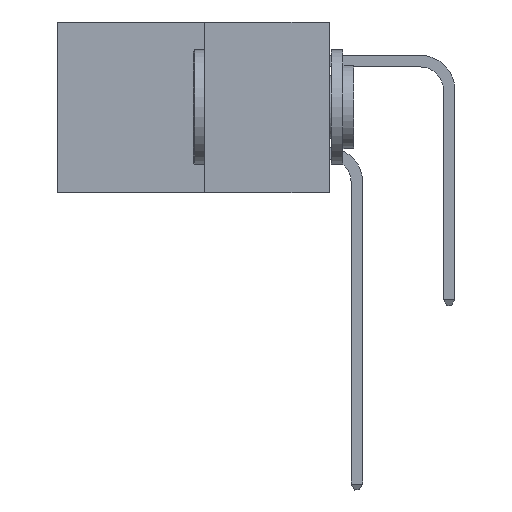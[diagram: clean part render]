
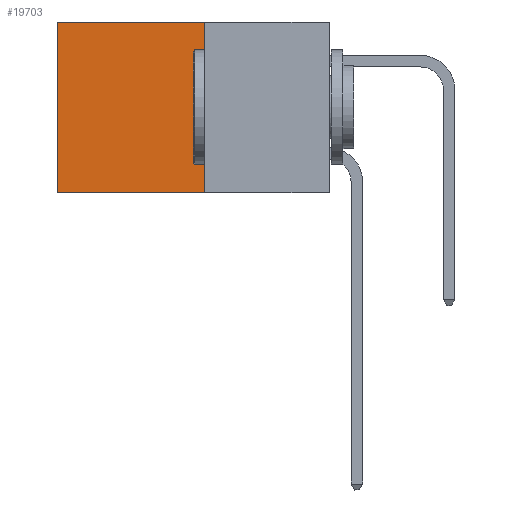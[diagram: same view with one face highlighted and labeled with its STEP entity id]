
A CAD part, left-side view. The second image highlights one B-rep face of the part: STEP entity #19703.
In plain terms, the highlighted planar face has unit normal (-1, 0, 0).
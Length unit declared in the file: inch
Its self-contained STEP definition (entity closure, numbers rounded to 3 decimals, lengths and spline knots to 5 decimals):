
#327 = CARTESIAN_POINT ( 'NONE',  ( 0.277, 0.27, -0.37 ) ) ;
#376 = CARTESIAN_POINT ( 'NONE',  ( 0.277, 0.27, -0.37 ) ) ;
#465 = CARTESIAN_POINT ( 'NONE',  ( 0.277, 0.27, -0.37 ) ) ;
#513 = AXIS2_PLACEMENT_3D ( 'NONE', #376, #20575, #9628 ) ;
#667 = DIRECTION ( 'NONE',  ( 0., 0., -1. ) ) ;
#1044 = VERTEX_POINT ( 'NONE', #13403 ) ;
#1388 = ORIENTED_EDGE ( 'NONE', *, *, #18385, .F. ) ;
#2605 = CARTESIAN_POINT ( 'NONE',  ( 0.277, 0.59, -0.37 ) ) ;
#6159 = CARTESIAN_POINT ( 'NONE',  ( 0.277, 0.27, -0.37 ) ) ;
#6398 = EDGE_CURVE ( 'NONE', #1044, #16911, #11830, .T. ) ;
#6986 = CARTESIAN_POINT ( 'NONE',  ( 0.277, 0.27, 0. ) ) ;
#7128 = EDGE_LOOP ( 'NONE', ( #21407, #22601, #1388, #15253 ) ) ;
#7780 = PLANE ( 'NONE',  #513 ) ;
#7942 = VERTEX_POINT ( 'NONE', #465 ) ;
#8034 = DIRECTION ( 'NONE',  ( 0., 0., -1. ) ) ;
#9628 = DIRECTION ( 'NONE',  ( 0., 0., -1. ) ) ;
#9882 = FACE_OUTER_BOUND ( 'NONE', #7128, .T. ) ;
#11097 = VERTEX_POINT ( 'NONE', #2605 ) ;
#11830 = LINE ( 'NONE', #6986, #21521 ) ;
#13124 = CARTESIAN_POINT ( 'NONE',  ( 0.277, 0.59, 0. ) ) ;
#13269 = VECTOR ( 'NONE', #16856, 39.37008 ) ;
#13403 = CARTESIAN_POINT ( 'NONE',  ( 0.277, 0.27, 0. ) ) ;
#14518 = EDGE_CURVE ( 'NONE', #7942, #11097, #18119, .T. ) ;
#15253 = ORIENTED_EDGE ( 'NONE', *, *, #6398, .T. ) ;
#16264 = LINE ( 'NONE', #17172, #19968 ) ;
#16856 = DIRECTION ( 'NONE',  ( 0., 1., 0. ) ) ;
#16911 = VERTEX_POINT ( 'NONE', #13124 ) ;
#17056 = VECTOR ( 'NONE', #667, 39.37008 ) ;
#17172 = CARTESIAN_POINT ( 'NONE',  ( 0.277, 0.59, -0.37 ) ) ;
#17697 = EDGE_CURVE ( 'NONE', #16911, #11097, #16264, .T. ) ;
#18119 = LINE ( 'NONE', #327, #13269 ) ;
#18385 = EDGE_CURVE ( 'NONE', #1044, #7942, #21906, .T. ) ;
#19703 = ADVANCED_FACE ( 'NONE', ( #9882 ), #7780, .F. ) ;
#19793 = DIRECTION ( 'NONE',  ( 0., 1., 0. ) ) ;
#19968 = VECTOR ( 'NONE', #8034, 39.37008 ) ;
#20575 = DIRECTION ( 'NONE',  ( 1., 0., 0. ) ) ;
#21407 = ORIENTED_EDGE ( 'NONE', *, *, #17697, .T. ) ;
#21521 = VECTOR ( 'NONE', #19793, 39.37008 ) ;
#21906 = LINE ( 'NONE', #6159, #17056 ) ;
#22601 = ORIENTED_EDGE ( 'NONE', *, *, #14518, .F. ) ;
